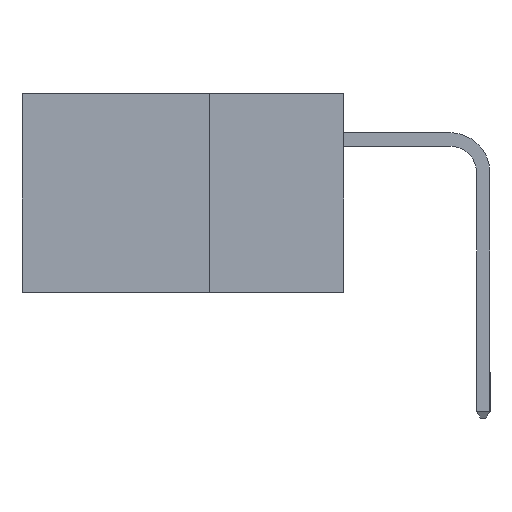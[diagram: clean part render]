
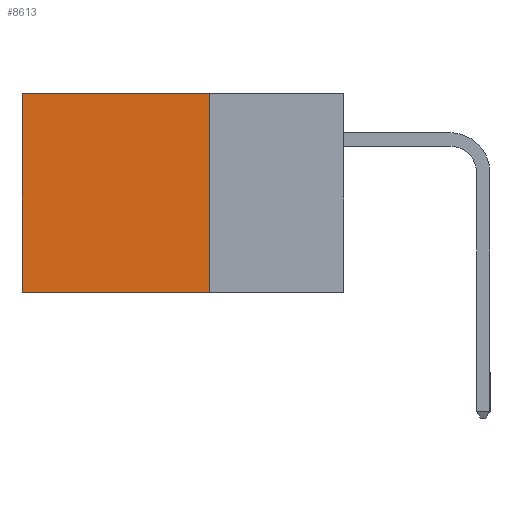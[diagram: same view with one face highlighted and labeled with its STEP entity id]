
A CAD part, left-side view. The second image highlights one B-rep face of the part: STEP entity #8613.
In plain terms, the highlighted planar face has unit normal (-1, 0, 0).
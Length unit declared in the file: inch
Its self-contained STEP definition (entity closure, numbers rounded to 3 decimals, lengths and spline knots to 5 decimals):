
#164 = LINE ( 'NONE', #14844, #9548 ) ;
#1073 = DIRECTION ( 'NONE',  ( 0., 0., -1. ) ) ;
#1209 = EDGE_LOOP ( 'NONE', ( #9134, #15478, #8546, #9386 ) ) ;
#3014 = EDGE_CURVE ( 'NONE', #18581, #16598, #15754, .T. ) ;
#3720 = VECTOR ( 'NONE', #6841, 39.37008 ) ;
#3739 = LINE ( 'NONE', #11662, #3720 ) ;
#4141 = VECTOR ( 'NONE', #15035, 39.37008 ) ;
#5614 = CARTESIAN_POINT ( 'NONE',  ( 0.2615, 0.25, -0.37 ) ) ;
#6107 = FACE_OUTER_BOUND ( 'NONE', #1209, .T. ) ;
#6841 = DIRECTION ( 'NONE',  ( 0., 1., 0. ) ) ;
#7035 = VECTOR ( 'NONE', #1073, 39.37008 ) ;
#7931 = VERTEX_POINT ( 'NONE', #16346 ) ;
#8546 = ORIENTED_EDGE ( 'NONE', *, *, #3014, .F. ) ;
#8596 = LINE ( 'NONE', #5614, #4141 ) ;
#8613 = ADVANCED_FACE ( 'NONE', ( #6107 ), #12419, .F. ) ;
#9134 = ORIENTED_EDGE ( 'NONE', *, *, #19961, .T. ) ;
#9386 = ORIENTED_EDGE ( 'NONE', *, *, #17175, .T. ) ;
#9548 = VECTOR ( 'NONE', #14527, 39.37008 ) ;
#10712 = CARTESIAN_POINT ( 'NONE',  ( 0.2615, 0.25, -0.37 ) ) ;
#11662 = CARTESIAN_POINT ( 'NONE',  ( 0.2615, 0.25, 0. ) ) ;
#11795 = CARTESIAN_POINT ( 'NONE',  ( 0.2615, 0.25, -0.37 ) ) ;
#12022 = EDGE_CURVE ( 'NONE', #16598, #12117, #8596, .T. ) ;
#12117 = VERTEX_POINT ( 'NONE', #20303 ) ;
#12315 = DIRECTION ( 'NONE',  ( 0., 0., -1. ) ) ;
#12419 = PLANE ( 'NONE',  #13010 ) ;
#13010 = AXIS2_PLACEMENT_3D ( 'NONE', #19078, #18877, #12315 ) ;
#14527 = DIRECTION ( 'NONE',  ( 0., 0., -1. ) ) ;
#14844 = CARTESIAN_POINT ( 'NONE',  ( 0.2615, 0.6, -0.37 ) ) ;
#15035 = DIRECTION ( 'NONE',  ( 0., 1., 0. ) ) ;
#15478 = ORIENTED_EDGE ( 'NONE', *, *, #12022, .F. ) ;
#15754 = LINE ( 'NONE', #10712, #7035 ) ;
#16346 = CARTESIAN_POINT ( 'NONE',  ( 0.2615, 0.6, 0. ) ) ;
#16598 = VERTEX_POINT ( 'NONE', #11795 ) ;
#17175 = EDGE_CURVE ( 'NONE', #18581, #7931, #3739, .T. ) ;
#18581 = VERTEX_POINT ( 'NONE', #18956 ) ;
#18877 = DIRECTION ( 'NONE',  ( 1., 0., 0. ) ) ;
#18956 = CARTESIAN_POINT ( 'NONE',  ( 0.2615, 0.25, 0. ) ) ;
#19078 = CARTESIAN_POINT ( 'NONE',  ( 0.2615, 0.25, -0.37 ) ) ;
#19961 = EDGE_CURVE ( 'NONE', #7931, #12117, #164, .T. ) ;
#20303 = CARTESIAN_POINT ( 'NONE',  ( 0.2615, 0.6, -0.37 ) ) ;
